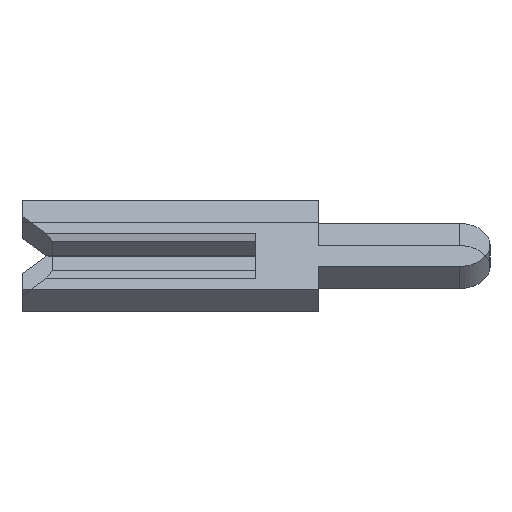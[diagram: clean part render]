
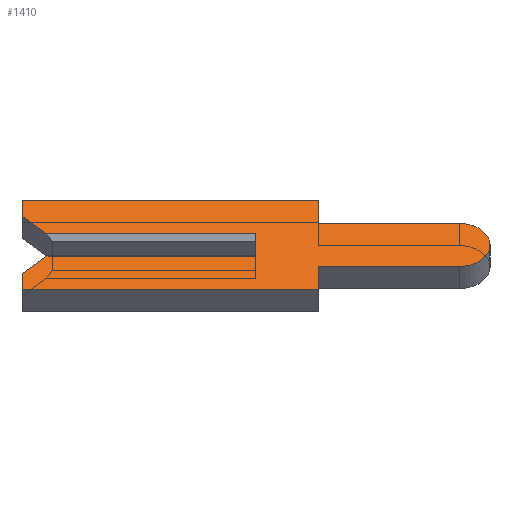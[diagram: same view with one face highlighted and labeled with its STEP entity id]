
A CAD part, left-side view. The second image highlights one B-rep face of the part: STEP entity #1410.
In plain terms, the highlighted face is planar.
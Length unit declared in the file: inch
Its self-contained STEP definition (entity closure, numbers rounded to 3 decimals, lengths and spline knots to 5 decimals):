
#1 = CARTESIAN_POINT ( 'NONE',  ( -0.01, -0.04, 0.0195 ) ) ;
#107 = ORIENTED_EDGE ( 'NONE', *, *, #626, .F. ) ;
#110 = CARTESIAN_POINT ( 'NONE',  ( -0.01, -0.04, -0.0195 ) ) ;
#138 = DIRECTION ( 'NONE',  ( 0., 0., -1. ) ) ;
#149 = VERTEX_POINT ( 'NONE', #1938 ) ;
#188 = CARTESIAN_POINT ( 'NONE',  ( -0.01, 0., -0.01 ) ) ;
#197 = ORIENTED_EDGE ( 'NONE', *, *, #640, .F. ) ;
#202 = CARTESIAN_POINT ( 'NONE',  ( -0.01, -0.04, 0.0195 ) ) ;
#239 = CARTESIAN_POINT ( 'NONE',  ( -0.01, 0.15, 0.04 ) ) ;
#284 = FACE_OUTER_BOUND ( 'NONE', #1832, .T. ) ;
#291 = DIRECTION ( 'NONE',  ( 0., 0.707, 0.707 ) ) ;
#332 = CARTESIAN_POINT ( 'NONE',  ( -0.01, 0.15, 0.04 ) ) ;
#346 = CARTESIAN_POINT ( 'NONE',  ( -0.01, 0.15, -0.04 ) ) ;
#352 = VERTEX_POINT ( 'NONE', #2174 ) ;
#360 = CARTESIAN_POINT ( 'NONE',  ( -0.01, 0.15, 0.026 ) ) ;
#384 = VERTEX_POINT ( 'NONE', #188 ) ;
#430 = VECTOR ( 'NONE', #2716, 39.37008 ) ;
#433 = CARTESIAN_POINT ( 'NONE',  ( -0.01, 0.15, 0.01 ) ) ;
#434 = EDGE_CURVE ( 'NONE', #384, #2552, #2737, .T. ) ;
#452 = AXIS2_PLACEMENT_3D ( 'NONE', #2476, #2003, #2519 ) ;
#455 = DIRECTION ( 'NONE',  ( 0., 0., 1. ) ) ;
#489 = CARTESIAN_POINT ( 'NONE',  ( -0.01, 0.1305, -0.0065 ) ) ;
#497 = LINE ( 'NONE', #2435, #2757 ) ;
#502 = VECTOR ( 'NONE', #2999, 39.37008 ) ;
#624 = VERTEX_POINT ( 'NONE', #698 ) ;
#626 = EDGE_CURVE ( 'NONE', #149, #352, #497, .T. ) ;
#640 = EDGE_CURVE ( 'NONE', #2626, #1357, #2379, .T. ) ;
#652 = VECTOR ( 'NONE', #455, 39.37008 ) ;
#683 = EDGE_CURVE ( 'NONE', #2872, #898, #1751, .T. ) ;
#698 = CARTESIAN_POINT ( 'NONE',  ( -0.01, -0.04, -0.0195 ) ) ;
#718 = LINE ( 'NONE', #1569, #2001 ) ;
#748 = ORIENTED_EDGE ( 'NONE', *, *, #811, .F. ) ;
#752 = LINE ( 'NONE', #110, #1959 ) ;
#789 = CARTESIAN_POINT ( 'NONE',  ( -0.01, 0.134, -0.01 ) ) ;
#811 = EDGE_CURVE ( 'NONE', #352, #1793, #1327, .T. ) ;
#831 = CARTESIAN_POINT ( 'NONE',  ( -0.01, -0.04, -0.04 ) ) ;
#853 = CARTESIAN_POINT ( 'NONE',  ( -0.01, 0., 0.01 ) ) ;
#898 = VERTEX_POINT ( 'NONE', #1 ) ;
#936 = DIRECTION ( 'NONE',  ( 0., 0., 1. ) ) ;
#966 = ORIENTED_EDGE ( 'NONE', *, *, #2665, .F. ) ;
#1020 = VECTOR ( 'NONE', #1511, 39.37008 ) ;
#1056 = LINE ( 'NONE', #332, #1846 ) ;
#1070 = VECTOR ( 'NONE', #2951, 39.37008 ) ;
#1090 = DIRECTION ( 'NONE',  ( 0., -1., 0. ) ) ;
#1100 = DIRECTION ( 'NONE',  ( 0., 1., 0. ) ) ;
#1162 = CARTESIAN_POINT ( 'NONE',  ( -0.01, -0.04, 0.04 ) ) ;
#1250 = PLANE ( 'NONE',  #452 ) ;
#1324 = CARTESIAN_POINT ( 'NONE',  ( -0.01, -0.1305, -0.01 ) ) ;
#1327 = LINE ( 'NONE', #489, #1020 ) ;
#1357 = VERTEX_POINT ( 'NONE', #239 ) ;
#1387 = ORIENTED_EDGE ( 'NONE', *, *, #683, .F. ) ;
#1406 = VECTOR ( 'NONE', #1533, 39.37008 ) ;
#1410 = ADVANCED_FACE ( 'NONE', ( #284 ), #1250, .F. ) ;
#1511 = DIRECTION ( 'NONE',  ( 0., -0.707, 0.707 ) ) ;
#1533 = DIRECTION ( 'NONE',  ( 0., -1., 0. ) ) ;
#1560 = EDGE_CURVE ( 'NONE', #898, #2308, #2428, .T. ) ;
#1569 = CARTESIAN_POINT ( 'NONE',  ( -0.01, -0.04, -0.04 ) ) ;
#1634 = ORIENTED_EDGE ( 'NONE', *, *, #434, .F. ) ;
#1638 = CARTESIAN_POINT ( 'NONE',  ( -0.01, -0.1305, 0. ) ) ;
#1645 = VECTOR ( 'NONE', #2628, 39.37008 ) ;
#1671 = VERTEX_POINT ( 'NONE', #1780 ) ;
#1687 = LINE ( 'NONE', #1324, #1406 ) ;
#1707 = EDGE_CURVE ( 'NONE', #624, #2622, #718, .T. ) ;
#1751 = LINE ( 'NONE', #1162, #1070 ) ;
#1780 = CARTESIAN_POINT ( 'NONE',  ( -0.01, 0.134, 0.01 ) ) ;
#1793 = VERTEX_POINT ( 'NONE', #789 ) ;
#1832 = EDGE_LOOP ( 'NONE', ( #2419, #1634, #2339, #748, #107, #2833, #2505, #966, #2994, #3074, #1387, #2305, #197, #3068 ) ) ;
#1846 = VECTOR ( 'NONE', #1090, 39.37008 ) ;
#1933 = EDGE_CURVE ( 'NONE', #1793, #384, #1687, .T. ) ;
#1938 = CARTESIAN_POINT ( 'NONE',  ( -0.01, 0.15, -0.04 ) ) ;
#1959 = VECTOR ( 'NONE', #1100, 39.37008 ) ;
#1983 = VERTEX_POINT ( 'NONE', #2278 ) ;
#2001 = VECTOR ( 'NONE', #2540, 39.37008 ) ;
#2003 = DIRECTION ( 'NONE',  ( 1., 0., 0. ) ) ;
#2080 = EDGE_CURVE ( 'NONE', #1671, #2626, #2921, .T. ) ;
#2153 = DIRECTION ( 'NONE',  ( 1., 0., 0. ) ) ;
#2168 = DIRECTION ( 'NONE',  ( 0., -1., 0. ) ) ;
#2174 = CARTESIAN_POINT ( 'NONE',  ( -0.01, 0.15, -0.026 ) ) ;
#2272 = EDGE_CURVE ( 'NONE', #1357, #2872, #1056, .T. ) ;
#2278 = CARTESIAN_POINT ( 'NONE',  ( -0.01, -0.1305, -0.0195 ) ) ;
#2296 = EDGE_CURVE ( 'NONE', #2622, #149, #2719, .T. ) ;
#2305 = ORIENTED_EDGE ( 'NONE', *, *, #2272, .F. ) ;
#2308 = VERTEX_POINT ( 'NONE', #3115 ) ;
#2315 = CARTESIAN_POINT ( 'NONE',  ( -0.01, 0.1305, 0.0065 ) ) ;
#2330 = CARTESIAN_POINT ( 'NONE',  ( -0.01, -0.04, 0.04 ) ) ;
#2339 = ORIENTED_EDGE ( 'NONE', *, *, #1933, .F. ) ;
#2379 = LINE ( 'NONE', #2981, #502 ) ;
#2419 = ORIENTED_EDGE ( 'NONE', *, *, #3052, .T. ) ;
#2428 = LINE ( 'NONE', #202, #430 ) ;
#2435 = CARTESIAN_POINT ( 'NONE',  ( -0.01, 0.15, -0.026 ) ) ;
#2476 = CARTESIAN_POINT ( 'NONE',  ( -0.01, -0.1305, 0. ) ) ;
#2505 = ORIENTED_EDGE ( 'NONE', *, *, #1707, .F. ) ;
#2519 = DIRECTION ( 'NONE',  ( 0., 0., -1. ) ) ;
#2524 = CIRCLE ( 'NONE', #3007, 0.0195 ) ;
#2540 = DIRECTION ( 'NONE',  ( 0., 0., -1. ) ) ;
#2552 = VERTEX_POINT ( 'NONE', #853 ) ;
#2622 = VERTEX_POINT ( 'NONE', #831 ) ;
#2626 = VERTEX_POINT ( 'NONE', #360 ) ;
#2628 = DIRECTION ( 'NONE',  ( 0., 1., 0. ) ) ;
#2665 = EDGE_CURVE ( 'NONE', #1983, #624, #752, .T. ) ;
#2716 = DIRECTION ( 'NONE',  ( 0., -1., 0. ) ) ;
#2719 = LINE ( 'NONE', #346, #1645 ) ;
#2737 = LINE ( 'NONE', #2742, #652 ) ;
#2742 = CARTESIAN_POINT ( 'NONE',  ( -0.01, 0., 0.0065 ) ) ;
#2757 = VECTOR ( 'NONE', #936, 39.37008 ) ;
#2833 = ORIENTED_EDGE ( 'NONE', *, *, #2296, .F. ) ;
#2859 = EDGE_CURVE ( 'NONE', #2308, #1983, #2524, .T. ) ;
#2872 = VERTEX_POINT ( 'NONE', #2330 ) ;
#2921 = LINE ( 'NONE', #2315, #3058 ) ;
#2951 = DIRECTION ( 'NONE',  ( 0., 0., -1. ) ) ;
#2965 = LINE ( 'NONE', #433, #3152 ) ;
#2981 = CARTESIAN_POINT ( 'NONE',  ( -0.01, 0.15, 0.026 ) ) ;
#2994 = ORIENTED_EDGE ( 'NONE', *, *, #2859, .F. ) ;
#2999 = DIRECTION ( 'NONE',  ( 0., 0., 1. ) ) ;
#3007 = AXIS2_PLACEMENT_3D ( 'NONE', #1638, #2153, #138 ) ;
#3052 = EDGE_CURVE ( 'NONE', #1671, #2552, #2965, .T. ) ;
#3058 = VECTOR ( 'NONE', #291, 39.37008 ) ;
#3068 = ORIENTED_EDGE ( 'NONE', *, *, #2080, .F. ) ;
#3074 = ORIENTED_EDGE ( 'NONE', *, *, #1560, .F. ) ;
#3115 = CARTESIAN_POINT ( 'NONE',  ( -0.01, -0.1305, 0.0195 ) ) ;
#3152 = VECTOR ( 'NONE', #2168, 39.37008 ) ;
